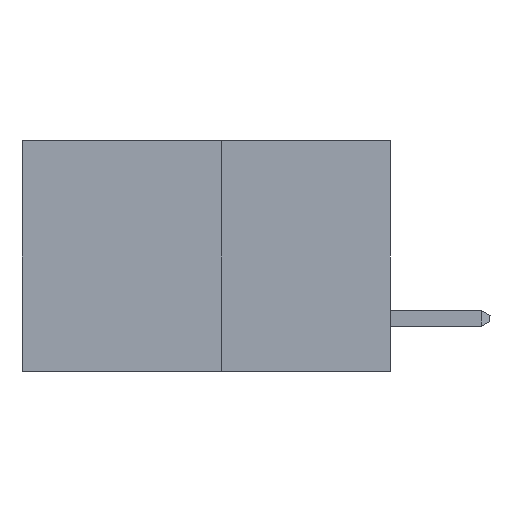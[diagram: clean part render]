
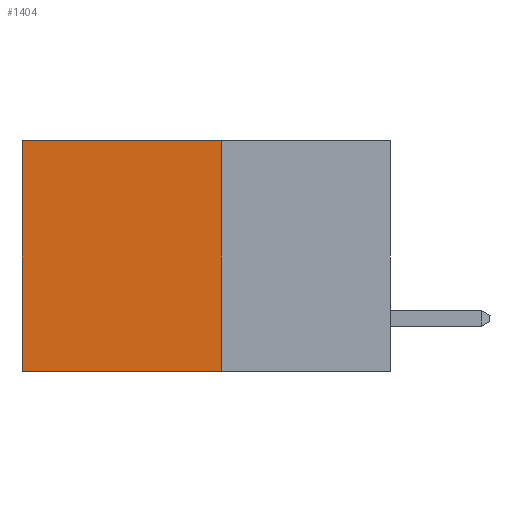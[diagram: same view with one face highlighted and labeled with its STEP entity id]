
A CAD part, left-side view. The second image highlights one B-rep face of the part: STEP entity #1404.
In plain terms, the highlighted planar face has unit normal (-1, 0, 0).
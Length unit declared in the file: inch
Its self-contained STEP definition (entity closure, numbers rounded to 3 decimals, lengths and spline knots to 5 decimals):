
#296 = VERTEX_POINT ( 'NONE', #10428 ) ;
#526 = VERTEX_POINT ( 'NONE', #10552 ) ;
#657 = CARTESIAN_POINT ( 'NONE',  ( 0.277, 0.27, -0.37 ) ) ;
#1197 = FACE_OUTER_BOUND ( 'NONE', #5171, .T. ) ;
#1404 = ADVANCED_FACE ( 'NONE', ( #1197 ), #7767, .F. ) ;
#1669 = EDGE_CURVE ( 'NONE', #7160, #526, #7987, .T. ) ;
#1870 = CARTESIAN_POINT ( 'NONE',  ( 0.277, 0.27, -0.37 ) ) ;
#2111 = LINE ( 'NONE', #2182, #10809 ) ;
#2182 = CARTESIAN_POINT ( 'NONE',  ( 0.277, 0.27, -0.37 ) ) ;
#2245 = VERTEX_POINT ( 'NONE', #4956 ) ;
#2381 = DIRECTION ( 'NONE',  ( 0., 0., -1. ) ) ;
#2432 = CARTESIAN_POINT ( 'NONE',  ( 0.277, 0.59, -0.37 ) ) ;
#2546 = VECTOR ( 'NONE', #4746, 39.37008 ) ;
#3433 = ORIENTED_EDGE ( 'NONE', *, *, #1669, .T. ) ;
#3490 = ORIENTED_EDGE ( 'NONE', *, *, #5569, .F. ) ;
#3584 = ORIENTED_EDGE ( 'NONE', *, *, #9062, .F. ) ;
#3618 = ORIENTED_EDGE ( 'NONE', *, *, #6021, .T. ) ;
#4468 = VECTOR ( 'NONE', #11148, 39.37008 ) ;
#4746 = DIRECTION ( 'NONE',  ( 0., 0., -1. ) ) ;
#4762 = LINE ( 'NONE', #6993, #4468 ) ;
#4848 = AXIS2_PLACEMENT_3D ( 'NONE', #1870, #7711, #7703 ) ;
#4956 = CARTESIAN_POINT ( 'NONE',  ( 0.277, 0.27, 0. ) ) ;
#5013 = LINE ( 'NONE', #657, #2546 ) ;
#5171 = EDGE_LOOP ( 'NONE', ( #3433, #3490, #3584, #3618 ) ) ;
#5569 = EDGE_CURVE ( 'NONE', #296, #526, #2111, .T. ) ;
#6021 = EDGE_CURVE ( 'NONE', #2245, #7160, #4762, .T. ) ;
#6993 = CARTESIAN_POINT ( 'NONE',  ( 0.277, 0.27, 0. ) ) ;
#7160 = VERTEX_POINT ( 'NONE', #8210 ) ;
#7514 = DIRECTION ( 'NONE',  ( 0., 1., 0. ) ) ;
#7703 = DIRECTION ( 'NONE',  ( 0., 0., -1. ) ) ;
#7711 = DIRECTION ( 'NONE',  ( 1., 0., 0. ) ) ;
#7767 = PLANE ( 'NONE',  #4848 ) ;
#7987 = LINE ( 'NONE', #2432, #8265 ) ;
#8210 = CARTESIAN_POINT ( 'NONE',  ( 0.277, 0.59, 0. ) ) ;
#8265 = VECTOR ( 'NONE', #2381, 39.37008 ) ;
#9062 = EDGE_CURVE ( 'NONE', #2245, #296, #5013, .T. ) ;
#10428 = CARTESIAN_POINT ( 'NONE',  ( 0.277, 0.27, -0.37 ) ) ;
#10552 = CARTESIAN_POINT ( 'NONE',  ( 0.277, 0.59, -0.37 ) ) ;
#10809 = VECTOR ( 'NONE', #7514, 39.37008 ) ;
#11148 = DIRECTION ( 'NONE',  ( 0., 1., 0. ) ) ;
